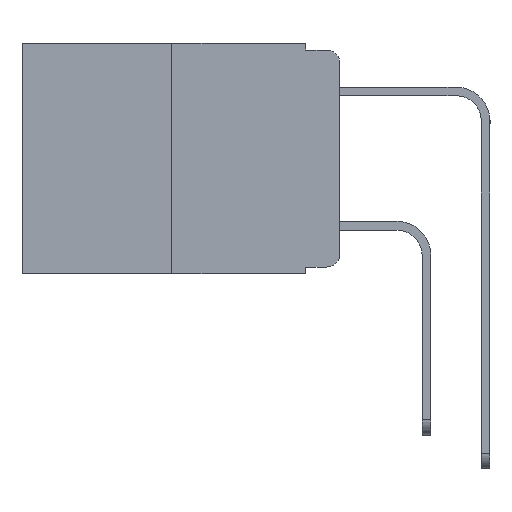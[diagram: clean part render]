
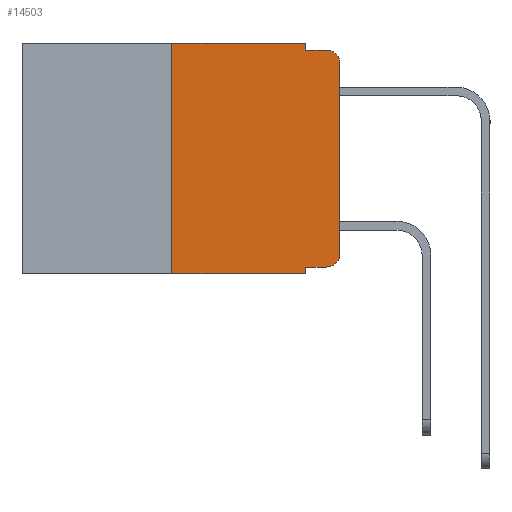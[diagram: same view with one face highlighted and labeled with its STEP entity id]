
A CAD part, left-side view. The second image highlights one B-rep face of the part: STEP entity #14503.
In plain terms, the highlighted planar face has unit normal (-1, 0, 0).
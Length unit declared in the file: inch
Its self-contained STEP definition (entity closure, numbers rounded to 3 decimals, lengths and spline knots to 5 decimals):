
#166 = EDGE_CURVE ( 'NONE', #3082, #3292, #13394, .T. ) ;
#548 = CARTESIAN_POINT ( 'NONE',  ( 0., 0., -0.03 ) ) ;
#973 = EDGE_CURVE ( 'NONE', #2334, #8803, #3817, .T. ) ;
#1006 = EDGE_CURVE ( 'NONE', #14207, #8803, #13754, .T. ) ;
#1100 = EDGE_CURVE ( 'NONE', #6718, #14207, #7746, .T. ) ;
#1128 = DIRECTION ( 'NONE',  ( 0., -1., 0. ) ) ;
#1332 = ORIENTED_EDGE ( 'NONE', *, *, #11179, .F. ) ;
#1724 = CARTESIAN_POINT ( 'NONE',  ( 0., 0., -0.313 ) ) ;
#1896 = CARTESIAN_POINT ( 'NONE',  ( 0., 0., 0. ) ) ;
#1908 = EDGE_CURVE ( 'NONE', #16138, #6718, #10624, .T. ) ;
#2329 = ORIENTED_EDGE ( 'NONE', *, *, #10291, .T. ) ;
#2334 = VERTEX_POINT ( 'NONE', #13672 ) ;
#2467 = AXIS2_PLACEMENT_3D ( 'NONE', #16897, #16285, #3037 ) ;
#3037 = DIRECTION ( 'NONE',  ( 0., 0., -1. ) ) ;
#3082 = VERTEX_POINT ( 'NONE', #14531 ) ;
#3194 = CARTESIAN_POINT ( 'NONE',  ( 0., 0.051, -0.01 ) ) ;
#3292 = VERTEX_POINT ( 'NONE', #11682 ) ;
#3294 = VECTOR ( 'NONE', #16569, 39.37008 ) ;
#3550 = CARTESIAN_POINT ( 'NONE',  ( 0., 0.25, -0.343 ) ) ;
#3817 = LINE ( 'NONE', #3194, #10653 ) ;
#4263 = VERTEX_POINT ( 'NONE', #3550 ) ;
#4377 = AXIS2_PLACEMENT_3D ( 'NONE', #15555, #16842, #8997 ) ;
#5235 = DIRECTION ( 'NONE',  ( 0., 0., 1. ) ) ;
#5604 = CARTESIAN_POINT ( 'NONE',  ( 0., 0.051, -0.343 ) ) ;
#6145 = ORIENTED_EDGE ( 'NONE', *, *, #1908, .T. ) ;
#6300 = VECTOR ( 'NONE', #9947, 39.37008 ) ;
#6341 = CARTESIAN_POINT ( 'NONE',  ( 0., 0.02, -0.01 ) ) ;
#6619 = LINE ( 'NONE', #7374, #3294 ) ;
#6718 = VERTEX_POINT ( 'NONE', #1724 ) ;
#6792 = CARTESIAN_POINT ( 'NONE',  ( 0., 0.02, -0.333 ) ) ;
#6920 = EDGE_LOOP ( 'NONE', ( #8077, #15082, #12017, #1332, #8891, #12430, #9311, #12841, #2329, #6145 ) ) ;
#7374 = CARTESIAN_POINT ( 'NONE',  ( 0., 0.051, 0. ) ) ;
#7746 = LINE ( 'NONE', #1896, #17759 ) ;
#8031 = AXIS2_PLACEMENT_3D ( 'NONE', #16029, #15742, #15737 ) ;
#8063 = LINE ( 'NONE', #8296, #17665 ) ;
#8077 = ORIENTED_EDGE ( 'NONE', *, *, #1100, .T. ) ;
#8089 = CARTESIAN_POINT ( 'NONE',  ( 0., 0.051, -0.333 ) ) ;
#8296 = CARTESIAN_POINT ( 'NONE',  ( 0., 0.473, -0.343 ) ) ;
#8422 = VECTOR ( 'NONE', #14982, 39.37008 ) ;
#8803 = VERTEX_POINT ( 'NONE', #6341 ) ;
#8869 = VECTOR ( 'NONE', #15961, 39.37008 ) ;
#8891 = ORIENTED_EDGE ( 'NONE', *, *, #166, .F. ) ;
#8997 = DIRECTION ( 'NONE',  ( 0., 0., -1. ) ) ;
#9311 = ORIENTED_EDGE ( 'NONE', *, *, #12391, .T. ) ;
#9606 = DIRECTION ( 'NONE',  ( 0., -1., 0. ) ) ;
#9947 = DIRECTION ( 'NONE',  ( 0., -1., 0. ) ) ;
#10271 = PLANE ( 'NONE',  #4377 ) ;
#10291 = EDGE_CURVE ( 'NONE', #14826, #16138, #12410, .T. ) ;
#10624 = CIRCLE ( 'NONE', #8031, 0.02 ) ;
#10653 = VECTOR ( 'NONE', #9606, 39.37008 ) ;
#10964 = CARTESIAN_POINT ( 'NONE',  ( 0., 0.051, -0.333 ) ) ;
#11016 = CARTESIAN_POINT ( 'NONE',  ( 0., 0.051, 0. ) ) ;
#11179 = EDGE_CURVE ( 'NONE', #3292, #2334, #6619, .T. ) ;
#11368 = VECTOR ( 'NONE', #13044, 39.37008 ) ;
#11682 = CARTESIAN_POINT ( 'NONE',  ( 0., 0.051, 0. ) ) ;
#11951 = LINE ( 'NONE', #11016, #8422 ) ;
#12017 = ORIENTED_EDGE ( 'NONE', *, *, #973, .F. ) ;
#12084 = EDGE_CURVE ( 'NONE', #4263, #3082, #14868, .T. ) ;
#12391 = EDGE_CURVE ( 'NONE', #4263, #12405, #8063, .T. ) ;
#12405 = VERTEX_POINT ( 'NONE', #5604 ) ;
#12410 = LINE ( 'NONE', #8089, #8869 ) ;
#12430 = ORIENTED_EDGE ( 'NONE', *, *, #12084, .F. ) ;
#12826 = CARTESIAN_POINT ( 'NONE',  ( 0., 0.473, 0. ) ) ;
#12841 = ORIENTED_EDGE ( 'NONE', *, *, #13839, .F. ) ;
#12952 = FACE_OUTER_BOUND ( 'NONE', #6920, .T. ) ;
#13044 = DIRECTION ( 'NONE',  ( 0., 0., 1. ) ) ;
#13394 = LINE ( 'NONE', #12826, #6300 ) ;
#13672 = CARTESIAN_POINT ( 'NONE',  ( 0., 0.051, -0.01 ) ) ;
#13754 = CIRCLE ( 'NONE', #2467, 0.02 ) ;
#13839 = EDGE_CURVE ( 'NONE', #14826, #12405, #11951, .T. ) ;
#14207 = VERTEX_POINT ( 'NONE', #548 ) ;
#14300 = CARTESIAN_POINT ( 'NONE',  ( 0., 0.25, 0. ) ) ;
#14503 = ADVANCED_FACE ( 'NONE', ( #12952 ), #10271, .F. ) ;
#14531 = CARTESIAN_POINT ( 'NONE',  ( 0., 0.25, 0. ) ) ;
#14826 = VERTEX_POINT ( 'NONE', #10964 ) ;
#14868 = LINE ( 'NONE', #14300, #11368 ) ;
#14982 = DIRECTION ( 'NONE',  ( 0., 0., -1. ) ) ;
#15082 = ORIENTED_EDGE ( 'NONE', *, *, #1006, .T. ) ;
#15555 = CARTESIAN_POINT ( 'NONE',  ( 0., 0.473, 0. ) ) ;
#15737 = DIRECTION ( 'NONE',  ( 0., 0., -1. ) ) ;
#15742 = DIRECTION ( 'NONE',  ( -1., 0., 0. ) ) ;
#15961 = DIRECTION ( 'NONE',  ( 0., -1., 0. ) ) ;
#16029 = CARTESIAN_POINT ( 'NONE',  ( 0., 0.02, -0.313 ) ) ;
#16138 = VERTEX_POINT ( 'NONE', #6792 ) ;
#16285 = DIRECTION ( 'NONE',  ( -1., 0., 0. ) ) ;
#16569 = DIRECTION ( 'NONE',  ( 0., 0., -1. ) ) ;
#16842 = DIRECTION ( 'NONE',  ( 1., 0., 0. ) ) ;
#16897 = CARTESIAN_POINT ( 'NONE',  ( 0., 0.02, -0.03 ) ) ;
#17665 = VECTOR ( 'NONE', #1128, 39.37008 ) ;
#17759 = VECTOR ( 'NONE', #5235, 39.37008 ) ;
